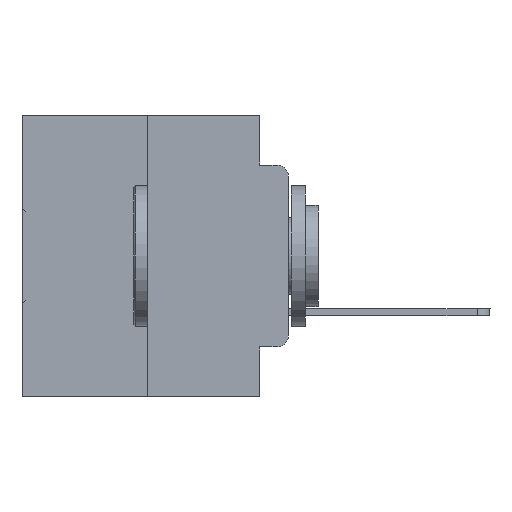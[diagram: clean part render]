
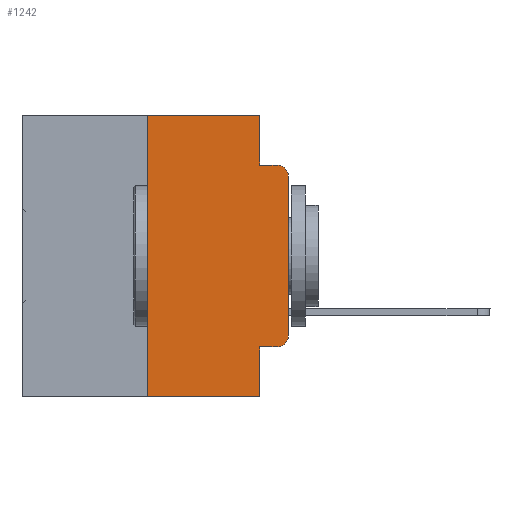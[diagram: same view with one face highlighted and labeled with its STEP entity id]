
A CAD part, left-side view. The second image highlights one B-rep face of the part: STEP entity #1242.
In plain terms, the highlighted planar face has unit normal (-1, 0, 0).
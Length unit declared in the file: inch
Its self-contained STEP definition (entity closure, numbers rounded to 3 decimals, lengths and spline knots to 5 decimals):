
#615 = ORIENTED_EDGE ( 'NONE', *, *, #18790, .F. ) ;
#649 = VERTEX_POINT ( 'NONE', #28245 ) ;
#1242 = ADVANCED_FACE ( 'NONE', ( #14676 ), #26238, .F. ) ;
#1416 = EDGE_CURVE ( 'NONE', #18488, #30105, #27296, .T. ) ;
#1478 = DIRECTION ( 'NONE',  ( 0., -1., 0. ) ) ;
#1918 = EDGE_CURVE ( 'NONE', #31656, #649, #16984, .T. ) ;
#2301 = AXIS2_PLACEMENT_3D ( 'NONE', #24087, #8996, #26632 ) ;
#3168 = CARTESIAN_POINT ( 'NONE',  ( 0., 0., -0.1085 ) ) ;
#3295 = VECTOR ( 'NONE', #1478, 39.37008 ) ;
#3301 = VECTOR ( 'NONE', #5379, 39.37008 ) ;
#3542 = CARTESIAN_POINT ( 'NONE',  ( 0., 0.25, 0. ) ) ;
#3696 = LINE ( 'NONE', #5266, #3301 ) ;
#3849 = DIRECTION ( 'NONE',  ( 1., 0., 0. ) ) ;
#5266 = CARTESIAN_POINT ( 'NONE',  ( 0., 0.051, -0.4115 ) ) ;
#5350 = VECTOR ( 'NONE', #16221, 39.37008 ) ;
#5379 = DIRECTION ( 'NONE',  ( 0., -1., 0. ) ) ;
#7630 = LINE ( 'NONE', #27440, #18678 ) ;
#8672 = ORIENTED_EDGE ( 'NONE', *, *, #27787, .T. ) ;
#8996 = DIRECTION ( 'NONE',  ( -1., 0., 0. ) ) ;
#9390 = EDGE_CURVE ( 'NONE', #25339, #26973, #3696, .T. ) ;
#9401 = CARTESIAN_POINT ( 'NONE',  ( 0., 0.051, 0. ) ) ;
#9502 = CARTESIAN_POINT ( 'NONE',  ( 0., 0.051, -0.4115 ) ) ;
#9765 = CARTESIAN_POINT ( 'NONE',  ( 0., 0., -0.3915 ) ) ;
#9766 = DIRECTION ( 'NONE',  ( 0., 0., -1. ) ) ;
#9999 = ORIENTED_EDGE ( 'NONE', *, *, #13026, .F. ) ;
#11337 = CARTESIAN_POINT ( 'NONE',  ( 0., 0.473, 0. ) ) ;
#12372 = DIRECTION ( 'NONE',  ( 0., 0., -1. ) ) ;
#13026 = EDGE_CURVE ( 'NONE', #17588, #25182, #27158, .T. ) ;
#13491 = CARTESIAN_POINT ( 'NONE',  ( 0., 0.25, 0. ) ) ;
#13725 = CARTESIAN_POINT ( 'NONE',  ( 0., 0.473, 0. ) ) ;
#13884 = DIRECTION ( 'NONE',  ( 0., 0., -1. ) ) ;
#14245 = AXIS2_PLACEMENT_3D ( 'NONE', #24607, #27469, #12372 ) ;
#14363 = CARTESIAN_POINT ( 'NONE',  ( 0., 0.051, 0. ) ) ;
#14626 = CARTESIAN_POINT ( 'NONE',  ( 0., 0.051, -0.5 ) ) ;
#14676 = FACE_OUTER_BOUND ( 'NONE', #30982, .T. ) ;
#16158 = VERTEX_POINT ( 'NONE', #9765 ) ;
#16221 = DIRECTION ( 'NONE',  ( 0., 0., 1. ) ) ;
#16984 = CIRCLE ( 'NONE', #2301, 0.02 ) ;
#17151 = ORIENTED_EDGE ( 'NONE', *, *, #1416, .T. ) ;
#17307 = VERTEX_POINT ( 'NONE', #23659 ) ;
#17588 = VERTEX_POINT ( 'NONE', #13491 ) ;
#17590 = CARTESIAN_POINT ( 'NONE',  ( 0., 0.473, -0.5 ) ) ;
#18432 = EDGE_CURVE ( 'NONE', #18488, #17588, #19956, .T. ) ;
#18463 = ORIENTED_EDGE ( 'NONE', *, *, #18432, .F. ) ;
#18488 = VERTEX_POINT ( 'NONE', #28635 ) ;
#18502 = ORIENTED_EDGE ( 'NONE', *, *, #26934, .F. ) ;
#18580 = ORIENTED_EDGE ( 'NONE', *, *, #9390, .T. ) ;
#18678 = VECTOR ( 'NONE', #25018, 39.37008 ) ;
#18790 = EDGE_CURVE ( 'NONE', #25339, #30105, #30207, .T. ) ;
#19820 = VECTOR ( 'NONE', #20237, 39.37008 ) ;
#19956 = LINE ( 'NONE', #3542, #5350 ) ;
#20237 = DIRECTION ( 'NONE',  ( 0., -1., 0. ) ) ;
#21013 = DIRECTION ( 'NONE',  ( 0., -1., 0. ) ) ;
#21888 = LINE ( 'NONE', #31666, #3295 ) ;
#22097 = DIRECTION ( 'NONE',  ( 0., 0., -1. ) ) ;
#23659 = CARTESIAN_POINT ( 'NONE',  ( 0., 0.051, -0.0885 ) ) ;
#23847 = LINE ( 'NONE', #9401, #25778 ) ;
#24087 = CARTESIAN_POINT ( 'NONE',  ( 0., 0.02, -0.1085 ) ) ;
#24607 = CARTESIAN_POINT ( 'NONE',  ( 0., 0.02, -0.3915 ) ) ;
#24644 = CARTESIAN_POINT ( 'NONE',  ( 0., 0.051, 0. ) ) ;
#24867 = ORIENTED_EDGE ( 'NONE', *, *, #1918, .T. ) ;
#25018 = DIRECTION ( 'NONE',  ( 0., 0., 1. ) ) ;
#25182 = VERTEX_POINT ( 'NONE', #14363 ) ;
#25206 = VECTOR ( 'NONE', #21013, 39.37008 ) ;
#25339 = VERTEX_POINT ( 'NONE', #9502 ) ;
#25778 = VECTOR ( 'NONE', #22097, 39.37008 ) ;
#26238 = PLANE ( 'NONE',  #27860 ) ;
#26524 = CIRCLE ( 'NONE', #14245, 0.02 ) ;
#26632 = DIRECTION ( 'NONE',  ( 0., 0., -1. ) ) ;
#26934 = EDGE_CURVE ( 'NONE', #17307, #649, #21888, .T. ) ;
#26973 = VERTEX_POINT ( 'NONE', #29235 ) ;
#27020 = VECTOR ( 'NONE', #9766, 39.37008 ) ;
#27158 = LINE ( 'NONE', #13725, #25206 ) ;
#27182 = EDGE_CURVE ( 'NONE', #25182, #17307, #23847, .T. ) ;
#27296 = LINE ( 'NONE', #17590, #19820 ) ;
#27440 = CARTESIAN_POINT ( 'NONE',  ( 0., 0., 0. ) ) ;
#27469 = DIRECTION ( 'NONE',  ( -1., 0., 0. ) ) ;
#27787 = EDGE_CURVE ( 'NONE', #16158, #31656, #7630, .T. ) ;
#27860 = AXIS2_PLACEMENT_3D ( 'NONE', #11337, #3849, #13884 ) ;
#28245 = CARTESIAN_POINT ( 'NONE',  ( 0., 0.02, -0.0885 ) ) ;
#28635 = CARTESIAN_POINT ( 'NONE',  ( 0., 0.25, -0.5 ) ) ;
#28937 = EDGE_CURVE ( 'NONE', #26973, #16158, #26524, .T. ) ;
#29235 = CARTESIAN_POINT ( 'NONE',  ( 0., 0.02, -0.4115 ) ) ;
#29631 = ORIENTED_EDGE ( 'NONE', *, *, #28937, .T. ) ;
#30073 = ORIENTED_EDGE ( 'NONE', *, *, #27182, .F. ) ;
#30105 = VERTEX_POINT ( 'NONE', #14626 ) ;
#30207 = LINE ( 'NONE', #24644, #27020 ) ;
#30982 = EDGE_LOOP ( 'NONE', ( #8672, #24867, #18502, #30073, #9999, #18463, #17151, #615, #18580, #29631 ) ) ;
#31656 = VERTEX_POINT ( 'NONE', #3168 ) ;
#31666 = CARTESIAN_POINT ( 'NONE',  ( 0., 0.051, -0.0885 ) ) ;
